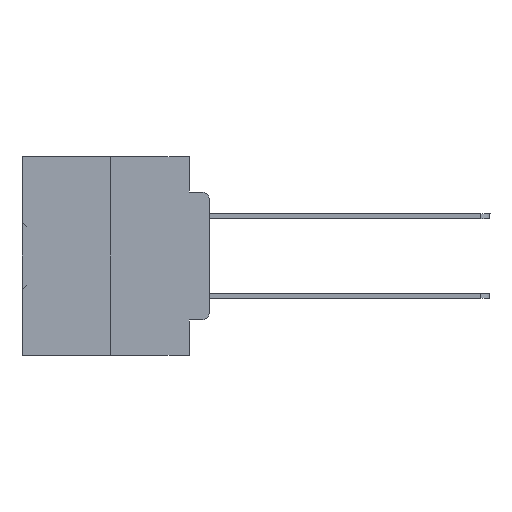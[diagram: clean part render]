
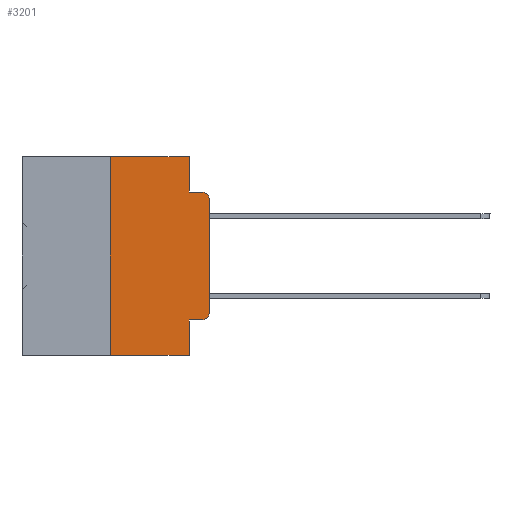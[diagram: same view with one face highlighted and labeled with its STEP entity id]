
A CAD part, left-side view. The second image highlights one B-rep face of the part: STEP entity #3201.
In plain terms, the highlighted planar face has unit normal (-1, 0, 0).
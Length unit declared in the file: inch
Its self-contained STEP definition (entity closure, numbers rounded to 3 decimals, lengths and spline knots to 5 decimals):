
#741 = ORIENTED_EDGE ( 'NONE', *, *, #20203, .T. ) ;
#798 = VERTEX_POINT ( 'NONE', #37891 ) ;
#1004 = VERTEX_POINT ( 'NONE', #28722 ) ;
#1064 = PLANE ( 'NONE',  #16869 ) ;
#1160 = CARTESIAN_POINT ( 'NONE',  ( 0., 0.051, -0.4115 ) ) ;
#1301 = ORIENTED_EDGE ( 'NONE', *, *, #39163, .F. ) ;
#1902 = VECTOR ( 'NONE', #28340, 39.37008 ) ;
#2054 = CARTESIAN_POINT ( 'NONE',  ( 0., 0.051, -0.0885 ) ) ;
#2807 = VERTEX_POINT ( 'NONE', #5419 ) ;
#3201 = ADVANCED_FACE ( 'NONE', ( #31335 ), #1064, .F. ) ;
#3488 = VECTOR ( 'NONE', #31436, 39.37008 ) ;
#3847 = CIRCLE ( 'NONE', #10977, 0.02 ) ;
#4103 = VERTEX_POINT ( 'NONE', #18318 ) ;
#4467 = CARTESIAN_POINT ( 'NONE',  ( 0., 0.051, -0.0885 ) ) ;
#4604 = CARTESIAN_POINT ( 'NONE',  ( 0., 0.02, -0.1085 ) ) ;
#5243 = ORIENTED_EDGE ( 'NONE', *, *, #11517, .F. ) ;
#5419 = CARTESIAN_POINT ( 'NONE',  ( 0., 0., -0.3915 ) ) ;
#6455 = DIRECTION ( 'NONE',  ( 0., 0., 1. ) ) ;
#6862 = CARTESIAN_POINT ( 'NONE',  ( 0., 0.25, 0. ) ) ;
#7256 = CARTESIAN_POINT ( 'NONE',  ( 0., 0.051, -0.4115 ) ) ;
#7882 = CARTESIAN_POINT ( 'NONE',  ( 0., 0., -0.1085 ) ) ;
#8211 = CARTESIAN_POINT ( 'NONE',  ( 0., 0.02, -0.3915 ) ) ;
#8276 = EDGE_LOOP ( 'NONE', ( #10678, #14957, #5243, #28630, #21769, #22920, #30924, #1301, #21015, #741 ) ) ;
#9147 = EDGE_CURVE ( 'NONE', #798, #4103, #35968, .T. ) ;
#9443 = EDGE_CURVE ( 'NONE', #2807, #25849, #21725, .T. ) ;
#9908 = DIRECTION ( 'NONE',  ( 0., 0., -1. ) ) ;
#10452 = DIRECTION ( 'NONE',  ( 0., 0., -1. ) ) ;
#10569 = LINE ( 'NONE', #31682, #28153 ) ;
#10678 = ORIENTED_EDGE ( 'NONE', *, *, #9443, .T. ) ;
#10977 = AXIS2_PLACEMENT_3D ( 'NONE', #8211, #32242, #26425 ) ;
#11375 = LINE ( 'NONE', #1160, #1902 ) ;
#11517 = EDGE_CURVE ( 'NONE', #37081, #26086, #30099, .T. ) ;
#13890 = CARTESIAN_POINT ( 'NONE',  ( 0., 0.051, 0. ) ) ;
#14957 = ORIENTED_EDGE ( 'NONE', *, *, #32814, .T. ) ;
#15559 = VECTOR ( 'NONE', #29259, 39.37008 ) ;
#16191 = AXIS2_PLACEMENT_3D ( 'NONE', #4604, #37884, #10452 ) ;
#16869 = AXIS2_PLACEMENT_3D ( 'NONE', #34359, #34096, #9908 ) ;
#18197 = LINE ( 'NONE', #13890, #30988 ) ;
#18318 = CARTESIAN_POINT ( 'NONE',  ( 0., 0.051, -0.5 ) ) ;
#19381 = VECTOR ( 'NONE', #6455, 39.37008 ) ;
#20078 = DIRECTION ( 'NONE',  ( 0., -1., 0. ) ) ;
#20203 = EDGE_CURVE ( 'NONE', #23698, #2807, #3847, .T. ) ;
#21015 = ORIENTED_EDGE ( 'NONE', *, *, #26130, .T. ) ;
#21720 = CARTESIAN_POINT ( 'NONE',  ( 0., 0.02, -0.4115 ) ) ;
#21725 = LINE ( 'NONE', #36453, #19381 ) ;
#21769 = ORIENTED_EDGE ( 'NONE', *, *, #22262, .F. ) ;
#22262 = EDGE_CURVE ( 'NONE', #25826, #1004, #23164, .T. ) ;
#22424 = DIRECTION ( 'NONE',  ( 0., 0., 1. ) ) ;
#22920 = ORIENTED_EDGE ( 'NONE', *, *, #30813, .F. ) ;
#23164 = LINE ( 'NONE', #25813, #15559 ) ;
#23698 = VERTEX_POINT ( 'NONE', #21720 ) ;
#25813 = CARTESIAN_POINT ( 'NONE',  ( 0., 0.473, 0. ) ) ;
#25826 = VERTEX_POINT ( 'NONE', #38532 ) ;
#25849 = VERTEX_POINT ( 'NONE', #7882 ) ;
#26086 = VERTEX_POINT ( 'NONE', #34329 ) ;
#26130 = EDGE_CURVE ( 'NONE', #34082, #23698, #11375, .T. ) ;
#26425 = DIRECTION ( 'NONE',  ( 0., 0., -1. ) ) ;
#28153 = VECTOR ( 'NONE', #38009, 39.37008 ) ;
#28340 = DIRECTION ( 'NONE',  ( 0., -1., 0. ) ) ;
#28630 = ORIENTED_EDGE ( 'NONE', *, *, #39039, .F. ) ;
#28722 = CARTESIAN_POINT ( 'NONE',  ( 0., 0.051, 0. ) ) ;
#29259 = DIRECTION ( 'NONE',  ( 0., -1., 0. ) ) ;
#29346 = CARTESIAN_POINT ( 'NONE',  ( 0., 0.473, -0.5 ) ) ;
#29831 = VECTOR ( 'NONE', #20078, 39.37008 ) ;
#30099 = LINE ( 'NONE', #4467, #3488 ) ;
#30813 = EDGE_CURVE ( 'NONE', #798, #25826, #37454, .T. ) ;
#30924 = ORIENTED_EDGE ( 'NONE', *, *, #9147, .T. ) ;
#30988 = VECTOR ( 'NONE', #38261, 39.37008 ) ;
#31335 = FACE_OUTER_BOUND ( 'NONE', #8276, .T. ) ;
#31436 = DIRECTION ( 'NONE',  ( 0., -1., 0. ) ) ;
#31682 = CARTESIAN_POINT ( 'NONE',  ( 0., 0.051, 0. ) ) ;
#32242 = DIRECTION ( 'NONE',  ( -1., 0., 0. ) ) ;
#32814 = EDGE_CURVE ( 'NONE', #25849, #26086, #39066, .T. ) ;
#34082 = VERTEX_POINT ( 'NONE', #7256 ) ;
#34096 = DIRECTION ( 'NONE',  ( 1., 0., 0. ) ) ;
#34329 = CARTESIAN_POINT ( 'NONE',  ( 0., 0.02, -0.0885 ) ) ;
#34359 = CARTESIAN_POINT ( 'NONE',  ( 0., 0.473, 0. ) ) ;
#35153 = VECTOR ( 'NONE', #22424, 39.37008 ) ;
#35968 = LINE ( 'NONE', #29346, #29831 ) ;
#36453 = CARTESIAN_POINT ( 'NONE',  ( 0., 0., 0. ) ) ;
#37081 = VERTEX_POINT ( 'NONE', #2054 ) ;
#37454 = LINE ( 'NONE', #6862, #35153 ) ;
#37884 = DIRECTION ( 'NONE',  ( -1., 0., 0. ) ) ;
#37891 = CARTESIAN_POINT ( 'NONE',  ( 0., 0.25, -0.5 ) ) ;
#38009 = DIRECTION ( 'NONE',  ( 0., 0., -1. ) ) ;
#38261 = DIRECTION ( 'NONE',  ( 0., 0., -1. ) ) ;
#38532 = CARTESIAN_POINT ( 'NONE',  ( 0., 0.25, 0. ) ) ;
#39039 = EDGE_CURVE ( 'NONE', #1004, #37081, #10569, .T. ) ;
#39066 = CIRCLE ( 'NONE', #16191, 0.02 ) ;
#39163 = EDGE_CURVE ( 'NONE', #34082, #4103, #18197, .T. ) ;
